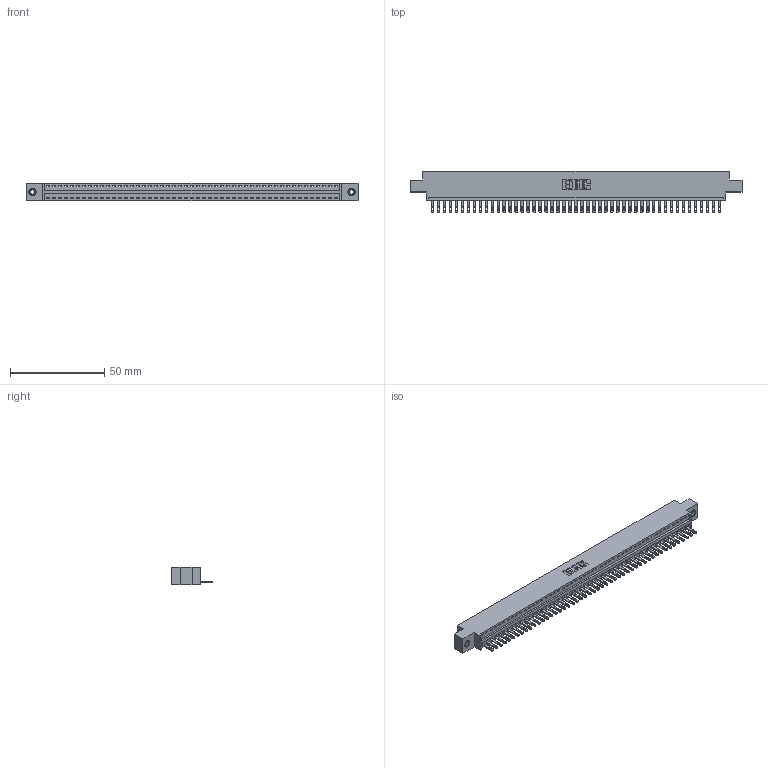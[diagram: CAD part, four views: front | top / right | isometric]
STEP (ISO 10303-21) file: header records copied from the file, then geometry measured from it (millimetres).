
FILE_DESCRIPTION (( 'STEP AP203' ), '1' );
FILE_NAME ('896-049-500-608.STEP', '2021-07-27T23:20:33', ( '' ), ( '' ), 'SwSTEP 2.0', 'SolidWorks 2020', '' );
FILE_SCHEMA (( 'CONFIG_CONTROL_DESIGN' ));
Length unit declared in the file: inch
Products named in the file (4): 345-292-001_345-293-100; 896-049-500-608; 345-250-001_345-250-003-102; 846 Part_0.170 Offset - 0.156 Dia-TI
Assembly tree (52 placements, depth 2):
  896-049-500-608
    846 Part_0.170 Offset - 0.156 Dia-TI
    345-292-001_345-293-100  x49
    345-250-001_345-250-003-102  x2
Bounding box: 176.15 x 21.84 x 9.4 mm (x, y, z)
Volume: 16778.8 mm3; surface area: 21343.2 mm2
Topology: 52 solids, 52 shells, 2832 faces, 8709 edges, 5798 vertices
Faces by surface type: plane 1778, cylinder 1038, cone 12, torus 4
Entity records: 30716 total; most frequent: CARTESIAN_POINT 5246, ORIENTED_EDGE 5222, DIRECTION 4647, EDGE_CURVE 2611, LINE 2259, VECTOR 2259, VERTEX_POINT 1736, AXIS2_PLACEMENT_3D 1194
